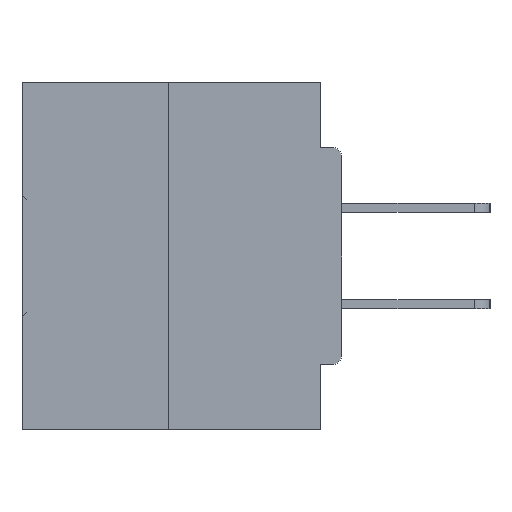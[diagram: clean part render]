
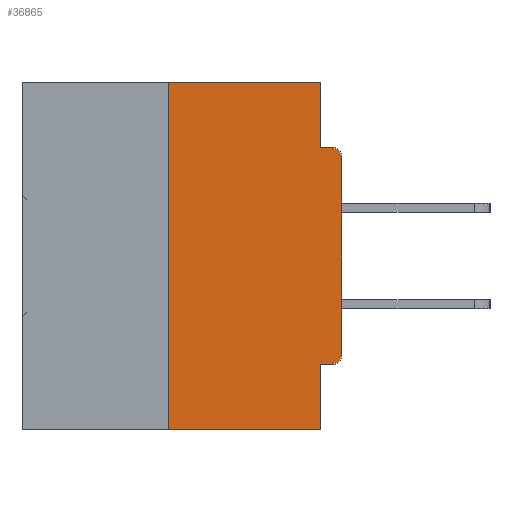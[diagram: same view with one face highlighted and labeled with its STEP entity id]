
A CAD part, left-side view. The second image highlights one B-rep face of the part: STEP entity #36865.
In plain terms, the highlighted planar face has unit normal (-1, 0, 0).
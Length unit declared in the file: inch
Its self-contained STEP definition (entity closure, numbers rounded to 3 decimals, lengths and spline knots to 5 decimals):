
#37 = DIRECTION ( 'NONE',  ( 0., 0., -1. ) ) ;
#246 = EDGE_CURVE ( 'NONE', #12024, #45329, #28108, .T. ) ;
#1692 = AXIS2_PLACEMENT_3D ( 'NONE', #33066, #29826, #43765 ) ;
#1734 = DIRECTION ( 'NONE',  ( 1., 0., 0. ) ) ;
#2530 = CARTESIAN_POINT ( 'NONE',  ( 0., 0.25, -0.5 ) ) ;
#4912 = EDGE_CURVE ( 'NONE', #42169, #37596, #38461, .T. ) ;
#5310 = CARTESIAN_POINT ( 'NONE',  ( 0., 0.031, -0.0935 ) ) ;
#5765 = DIRECTION ( 'NONE',  ( 0., 1., 0. ) ) ;
#5926 = CARTESIAN_POINT ( 'NONE',  ( 0., 0., -0.3915 ) ) ;
#5987 = VECTOR ( 'NONE', #36660, 39.37008 ) ;
#6887 = DIRECTION ( 'NONE',  ( 0., -1., 0. ) ) ;
#10453 = CARTESIAN_POINT ( 'NONE',  ( 0., 0.25, 0. ) ) ;
#10656 = EDGE_CURVE ( 'NONE', #18099, #11476, #38363, .T. ) ;
#10748 = VERTEX_POINT ( 'NONE', #14024 ) ;
#11476 = VERTEX_POINT ( 'NONE', #34470 ) ;
#12024 = VERTEX_POINT ( 'NONE', #5926 ) ;
#12704 = CARTESIAN_POINT ( 'NONE',  ( 0., 0.46, 0. ) ) ;
#13273 = DIRECTION ( 'NONE',  ( 0., -1., 0. ) ) ;
#13662 = DIRECTION ( 'NONE',  ( 0., 0., -1. ) ) ;
#13715 = VECTOR ( 'NONE', #40984, 39.37008 ) ;
#14024 = CARTESIAN_POINT ( 'NONE',  ( 0., 0.015, -0.4065 ) ) ;
#14160 = ORIENTED_EDGE ( 'NONE', *, *, #16889, .T. ) ;
#15957 = CIRCLE ( 'NONE', #1692, 0.015 ) ;
#16293 = CARTESIAN_POINT ( 'NONE',  ( 0., 0.25, 0. ) ) ;
#16889 = EDGE_CURVE ( 'NONE', #45329, #37143, #19335, .T. ) ;
#17483 = VECTOR ( 'NONE', #37, 39.37008 ) ;
#18099 = VERTEX_POINT ( 'NONE', #10453 ) ;
#18540 = ORIENTED_EDGE ( 'NONE', *, *, #40505, .F. ) ;
#18915 = ORIENTED_EDGE ( 'NONE', *, *, #38412, .F. ) ;
#19335 = CIRCLE ( 'NONE', #32031, 0.015 ) ;
#20106 = CARTESIAN_POINT ( 'NONE',  ( 0., 0., -0.1085 ) ) ;
#22275 = CARTESIAN_POINT ( 'NONE',  ( 0., 0.031, 0. ) ) ;
#22791 = VECTOR ( 'NONE', #6887, 39.37008 ) ;
#22807 = DIRECTION ( 'NONE',  ( 0., -1., 0. ) ) ;
#22878 = CARTESIAN_POINT ( 'NONE',  ( 0., 0., 0. ) ) ;
#23716 = LINE ( 'NONE', #34097, #34810 ) ;
#24533 = VERTEX_POINT ( 'NONE', #2530 ) ;
#24775 = CARTESIAN_POINT ( 'NONE',  ( 0., 0.015, -0.0935 ) ) ;
#25109 = EDGE_CURVE ( 'NONE', #24533, #18099, #34633, .T. ) ;
#27164 = ORIENTED_EDGE ( 'NONE', *, *, #4912, .F. ) ;
#27472 = DIRECTION ( 'NONE',  ( -1., 0., 0. ) ) ;
#27777 = EDGE_CURVE ( 'NONE', #10748, #12024, #15957, .T. ) ;
#28102 = CARTESIAN_POINT ( 'NONE',  ( 0., 0., -0.0935 ) ) ;
#28108 = LINE ( 'NONE', #22878, #40896 ) ;
#29606 = CARTESIAN_POINT ( 'NONE',  ( 0., 0.46, -0.5 ) ) ;
#29681 = EDGE_CURVE ( 'NONE', #24533, #37596, #44974, .T. ) ;
#29826 = DIRECTION ( 'NONE',  ( -1., 0., 0. ) ) ;
#30253 = LINE ( 'NONE', #22275, #5987 ) ;
#30450 = ORIENTED_EDGE ( 'NONE', *, *, #29681, .T. ) ;
#31346 = ORIENTED_EDGE ( 'NONE', *, *, #27777, .T. ) ;
#32031 = AXIS2_PLACEMENT_3D ( 'NONE', #34586, #27472, #13662 ) ;
#33066 = CARTESIAN_POINT ( 'NONE',  ( 0., 0.015, -0.3915 ) ) ;
#33386 = EDGE_LOOP ( 'NONE', ( #35992, #45356, #30450, #27164, #45198, #31346, #42225, #14160, #18915, #18540 ) ) ;
#34080 = DIRECTION ( 'NONE',  ( 0., 0., -1. ) ) ;
#34097 = CARTESIAN_POINT ( 'NONE',  ( 0., 0., -0.4065 ) ) ;
#34470 = CARTESIAN_POINT ( 'NONE',  ( 0., 0.031, 0. ) ) ;
#34508 = CARTESIAN_POINT ( 'NONE',  ( 0., 0.46, 0. ) ) ;
#34586 = CARTESIAN_POINT ( 'NONE',  ( 0., 0.015, -0.1085 ) ) ;
#34633 = LINE ( 'NONE', #16293, #13715 ) ;
#34810 = VECTOR ( 'NONE', #5765, 39.37008 ) ;
#35520 = VECTOR ( 'NONE', #22807, 39.37008 ) ;
#35992 = ORIENTED_EDGE ( 'NONE', *, *, #10656, .F. ) ;
#36086 = LINE ( 'NONE', #28102, #22791 ) ;
#36126 = VECTOR ( 'NONE', #13273, 39.37008 ) ;
#36630 = FACE_OUTER_BOUND ( 'NONE', #33386, .T. ) ;
#36660 = DIRECTION ( 'NONE',  ( 0., 0., -1. ) ) ;
#36865 = ADVANCED_FACE ( 'NONE', ( #36630 ), #44635, .F. ) ;
#37143 = VERTEX_POINT ( 'NONE', #24775 ) ;
#37596 = VERTEX_POINT ( 'NONE', #43837 ) ;
#38363 = LINE ( 'NONE', #34508, #36126 ) ;
#38412 = EDGE_CURVE ( 'NONE', #38867, #37143, #36086, .T. ) ;
#38461 = LINE ( 'NONE', #45598, #17483 ) ;
#38867 = VERTEX_POINT ( 'NONE', #5310 ) ;
#40505 = EDGE_CURVE ( 'NONE', #11476, #38867, #30253, .T. ) ;
#40896 = VECTOR ( 'NONE', #44232, 39.37008 ) ;
#40984 = DIRECTION ( 'NONE',  ( 0., 0., 1. ) ) ;
#42169 = VERTEX_POINT ( 'NONE', #44237 ) ;
#42225 = ORIENTED_EDGE ( 'NONE', *, *, #246, .T. ) ;
#43064 = AXIS2_PLACEMENT_3D ( 'NONE', #12704, #1734, #34080 ) ;
#43765 = DIRECTION ( 'NONE',  ( 0., 0., -1. ) ) ;
#43837 = CARTESIAN_POINT ( 'NONE',  ( 0., 0.031, -0.5 ) ) ;
#44232 = DIRECTION ( 'NONE',  ( 0., 0., 1. ) ) ;
#44237 = CARTESIAN_POINT ( 'NONE',  ( 0., 0.031, -0.4065 ) ) ;
#44635 = PLANE ( 'NONE',  #43064 ) ;
#44691 = EDGE_CURVE ( 'NONE', #10748, #42169, #23716, .T. ) ;
#44974 = LINE ( 'NONE', #29606, #35520 ) ;
#45198 = ORIENTED_EDGE ( 'NONE', *, *, #44691, .F. ) ;
#45329 = VERTEX_POINT ( 'NONE', #20106 ) ;
#45356 = ORIENTED_EDGE ( 'NONE', *, *, #25109, .F. ) ;
#45598 = CARTESIAN_POINT ( 'NONE',  ( 0., 0.031, -0.5 ) ) ;
